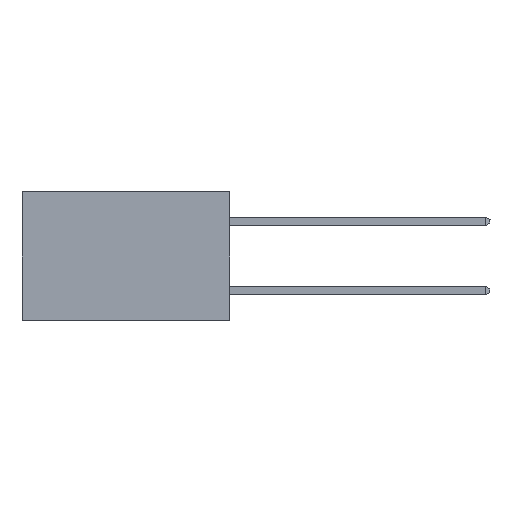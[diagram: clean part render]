
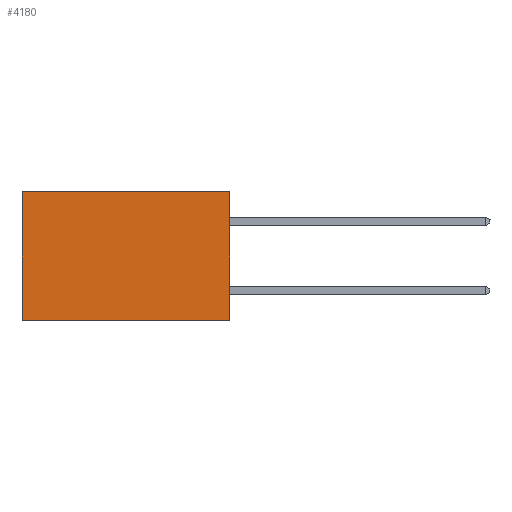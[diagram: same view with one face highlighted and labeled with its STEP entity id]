
A CAD part, left-side view. The second image highlights one B-rep face of the part: STEP entity #4180.
In plain terms, the highlighted planar face has unit normal (-1, 0, 0).
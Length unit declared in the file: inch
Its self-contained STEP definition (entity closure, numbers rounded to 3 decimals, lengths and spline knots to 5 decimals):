
#555 = ORIENTED_EDGE ( 'NONE', *, *, #5241, .F. ) ;
#867 = CARTESIAN_POINT ( 'NONE',  ( 0.2615, 0., 0. ) ) ;
#939 = LINE ( 'NONE', #867, #10534 ) ;
#1097 = VECTOR ( 'NONE', #11619, 39.37008 ) ;
#1109 = DIRECTION ( 'NONE',  ( 1., 0., 0. ) ) ;
#1172 = DIRECTION ( 'NONE',  ( 0., 0., -1. ) ) ;
#2193 = CARTESIAN_POINT ( 'NONE',  ( 0.2615, 0.6, 0. ) ) ;
#2822 = EDGE_CURVE ( 'NONE', #5873, #5319, #939, .T. ) ;
#3420 = VECTOR ( 'NONE', #3944, 39.37008 ) ;
#3663 = CARTESIAN_POINT ( 'NONE',  ( 0.2615, 0.6, -0.37 ) ) ;
#3944 = DIRECTION ( 'NONE',  ( 0., 1., 0. ) ) ;
#4180 = ADVANCED_FACE ( 'NONE', ( #9070 ), #10040, .F. ) ;
#4354 = VERTEX_POINT ( 'NONE', #8876 ) ;
#4776 = CARTESIAN_POINT ( 'NONE',  ( 0.2615, 0.6, -0.37 ) ) ;
#4926 = DIRECTION ( 'NONE',  ( 0., 1., 0. ) ) ;
#5241 = EDGE_CURVE ( 'NONE', #4354, #7528, #10060, .T. ) ;
#5319 = VERTEX_POINT ( 'NONE', #2193 ) ;
#5432 = AXIS2_PLACEMENT_3D ( 'NONE', #11097, #1109, #1172 ) ;
#5873 = VERTEX_POINT ( 'NONE', #10282 ) ;
#7272 = DIRECTION ( 'NONE',  ( 0., 0., -1. ) ) ;
#7528 = VERTEX_POINT ( 'NONE', #4776 ) ;
#7804 = ORIENTED_EDGE ( 'NONE', *, *, #12142, .F. ) ;
#8494 = CARTESIAN_POINT ( 'NONE',  ( 0.2615, 0., -0.37 ) ) ;
#8615 = LINE ( 'NONE', #3663, #1097 ) ;
#8876 = CARTESIAN_POINT ( 'NONE',  ( 0.2615, 0., -0.37 ) ) ;
#9029 = EDGE_CURVE ( 'NONE', #5319, #7528, #8615, .T. ) ;
#9070 = FACE_OUTER_BOUND ( 'NONE', #12002, .T. ) ;
#9277 = VECTOR ( 'NONE', #7272, 39.37008 ) ;
#9947 = CARTESIAN_POINT ( 'NONE',  ( 0.2615, 0., -0.37 ) ) ;
#10040 = PLANE ( 'NONE',  #5432 ) ;
#10060 = LINE ( 'NONE', #9947, #3420 ) ;
#10282 = CARTESIAN_POINT ( 'NONE',  ( 0.2615, 0., 0. ) ) ;
#10297 = LINE ( 'NONE', #8494, #9277 ) ;
#10534 = VECTOR ( 'NONE', #4926, 39.37008 ) ;
#10578 = ORIENTED_EDGE ( 'NONE', *, *, #2822, .T. ) ;
#11097 = CARTESIAN_POINT ( 'NONE',  ( 0.2615, 0., -0.37 ) ) ;
#11619 = DIRECTION ( 'NONE',  ( 0., 0., -1. ) ) ;
#11797 = ORIENTED_EDGE ( 'NONE', *, *, #9029, .T. ) ;
#12002 = EDGE_LOOP ( 'NONE', ( #11797, #555, #7804, #10578 ) ) ;
#12142 = EDGE_CURVE ( 'NONE', #5873, #4354, #10297, .T. ) ;
